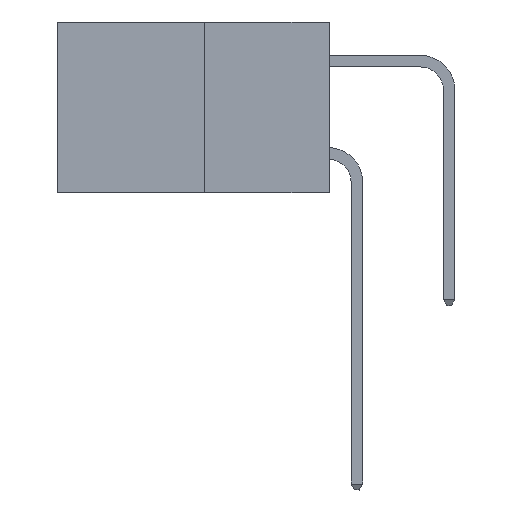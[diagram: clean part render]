
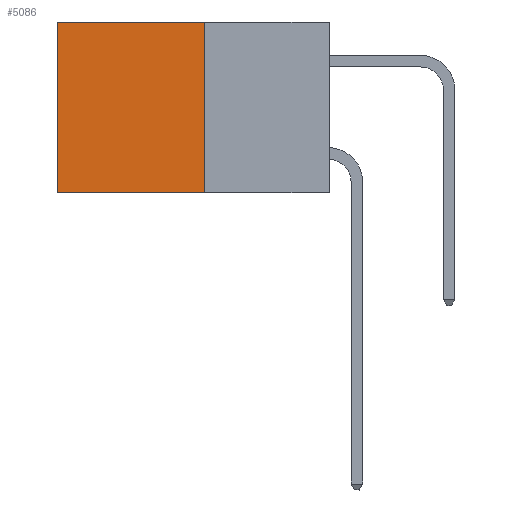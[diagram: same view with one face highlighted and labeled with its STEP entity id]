
A CAD part, left-side view. The second image highlights one B-rep face of the part: STEP entity #5086.
In plain terms, the highlighted planar face has unit normal (-1, 0, 0).
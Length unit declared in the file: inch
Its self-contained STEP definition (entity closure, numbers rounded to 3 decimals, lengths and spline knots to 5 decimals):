
#28 = DIRECTION ( 'NONE',  ( 0., 0., -1. ) ) ;
#223 = CARTESIAN_POINT ( 'NONE',  ( 0.277, 0.27, -0.37 ) ) ;
#568 = VERTEX_POINT ( 'NONE', #4682 ) ;
#901 = DIRECTION ( 'NONE',  ( 0., 1., 0. ) ) ;
#1374 = AXIS2_PLACEMENT_3D ( 'NONE', #8107, #5193, #5167 ) ;
#1676 = CARTESIAN_POINT ( 'NONE',  ( 0.277, 0.27, 0. ) ) ;
#1721 = DIRECTION ( 'NONE',  ( 0., 0., -1. ) ) ;
#1877 = ORIENTED_EDGE ( 'NONE', *, *, #6312, .F. ) ;
#2067 = EDGE_CURVE ( 'NONE', #8686, #7807, #6920, .T. ) ;
#2175 = CARTESIAN_POINT ( 'NONE',  ( 0.277, 0.27, -0.37 ) ) ;
#3434 = LINE ( 'NONE', #223, #5403 ) ;
#3586 = VECTOR ( 'NONE', #6519, 39.37008 ) ;
#3929 = EDGE_CURVE ( 'NONE', #7807, #4457, #5661, .T. ) ;
#4457 = VERTEX_POINT ( 'NONE', #8933 ) ;
#4682 = CARTESIAN_POINT ( 'NONE',  ( 0.277, 0.27, -0.37 ) ) ;
#5086 = ADVANCED_FACE ( 'NONE', ( #7772 ), #5825, .F. ) ;
#5167 = DIRECTION ( 'NONE',  ( 0., 0., -1. ) ) ;
#5193 = DIRECTION ( 'NONE',  ( 1., 0., 0. ) ) ;
#5244 = ORIENTED_EDGE ( 'NONE', *, *, #7404, .F. ) ;
#5309 = CARTESIAN_POINT ( 'NONE',  ( 0.277, 0.59, -0.37 ) ) ;
#5401 = VECTOR ( 'NONE', #1721, 39.37008 ) ;
#5403 = VECTOR ( 'NONE', #28, 39.37008 ) ;
#5661 = LINE ( 'NONE', #5309, #5401 ) ;
#5743 = ORIENTED_EDGE ( 'NONE', *, *, #2067, .T. ) ;
#5825 = PLANE ( 'NONE',  #1374 ) ;
#6312 = EDGE_CURVE ( 'NONE', #568, #4457, #7301, .T. ) ;
#6519 = DIRECTION ( 'NONE',  ( 0., 1., 0. ) ) ;
#6920 = LINE ( 'NONE', #8539, #8773 ) ;
#7094 = CARTESIAN_POINT ( 'NONE',  ( 0.277, 0.59, 0. ) ) ;
#7301 = LINE ( 'NONE', #2175, #3586 ) ;
#7404 = EDGE_CURVE ( 'NONE', #8686, #568, #3434, .T. ) ;
#7772 = FACE_OUTER_BOUND ( 'NONE', #8751, .T. ) ;
#7807 = VERTEX_POINT ( 'NONE', #7094 ) ;
#8107 = CARTESIAN_POINT ( 'NONE',  ( 0.277, 0.27, -0.37 ) ) ;
#8539 = CARTESIAN_POINT ( 'NONE',  ( 0.277, 0.27, 0. ) ) ;
#8686 = VERTEX_POINT ( 'NONE', #1676 ) ;
#8751 = EDGE_LOOP ( 'NONE', ( #9236, #1877, #5244, #5743 ) ) ;
#8773 = VECTOR ( 'NONE', #901, 39.37008 ) ;
#8933 = CARTESIAN_POINT ( 'NONE',  ( 0.277, 0.59, -0.37 ) ) ;
#9236 = ORIENTED_EDGE ( 'NONE', *, *, #3929, .T. ) ;
